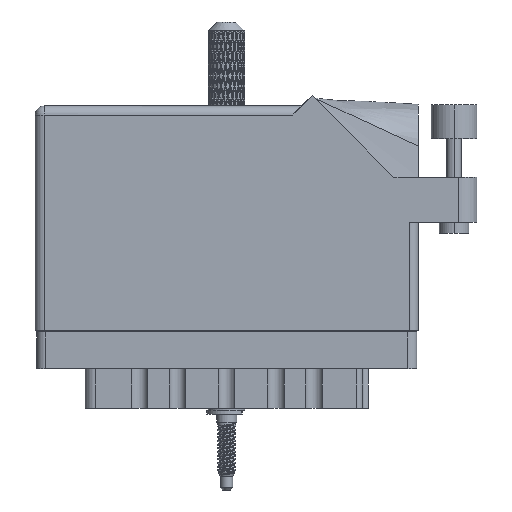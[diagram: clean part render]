
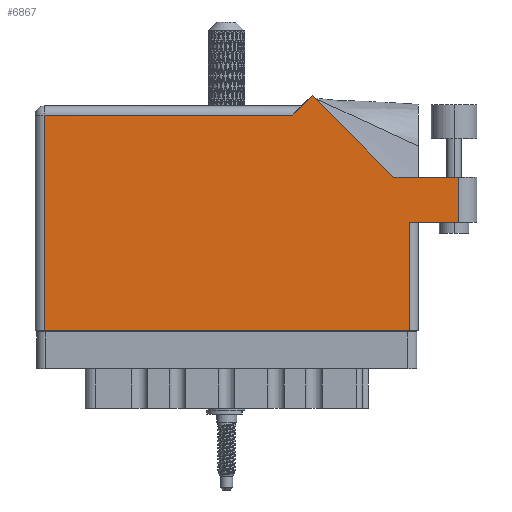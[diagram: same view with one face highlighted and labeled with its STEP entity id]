
A CAD part, front view. The second image highlights one B-rep face of the part: STEP entity #6867.
In plain terms, the highlighted face is planar.
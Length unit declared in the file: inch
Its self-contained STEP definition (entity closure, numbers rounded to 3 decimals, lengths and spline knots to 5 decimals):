
#557 = VERTEX_POINT ( 'NONE', #68809 ) ;
#1133 = CARTESIAN_POINT ( 'NONE',  ( 2.887, 0.737, 0. ) ) ;
#1200 = VECTOR ( 'NONE', #70098, 39.37008 ) ;
#2362 = LINE ( 'NONE', #81924, #64410 ) ;
#4994 = CARTESIAN_POINT ( 'NONE',  ( 0.062, 0., 0. ) ) ;
#5042 = CARTESIAN_POINT ( 'NONE',  ( 0.062, 0., 0. ) ) ;
#6867 = ADVANCED_FACE ( 'NONE', ( #55155 ), #33903, .F. ) ;
#9447 = DIRECTION ( 'NONE',  ( 0., 1., 0. ) ) ;
#10161 = LINE ( 'NONE', #42525, #63592 ) ;
#11218 = CARTESIAN_POINT ( 'NONE',  ( 1.757, 1.468, 0. ) ) ;
#14084 = EDGE_CURVE ( 'NONE', #20176, #74270, #48795, .T. ) ;
#15552 = VERTEX_POINT ( 'NONE', #52664 ) ;
#16435 = VECTOR ( 'NONE', #65704, 39.37008 ) ;
#17283 = CARTESIAN_POINT ( 'NONE',  ( 0., 1.53, 0. ) ) ;
#18609 = ORIENTED_EDGE ( 'NONE', *, *, #99939, .T. ) ;
#20176 = VERTEX_POINT ( 'NONE', #67402 ) ;
#20765 = VERTEX_POINT ( 'NONE', #1133 ) ;
#20951 = CARTESIAN_POINT ( 'NONE',  ( 0., 0., 0. ) ) ;
#24599 = DIRECTION ( 'NONE',  ( 0., 0., -1. ) ) ;
#25157 = LINE ( 'NONE', #73787, #16435 ) ;
#25183 = CARTESIAN_POINT ( 'NONE',  ( 2.44642, 1.044, 0. ) ) ;
#29127 = VERTEX_POINT ( 'NONE', #5042 ) ;
#30946 = EDGE_CURVE ( 'NONE', #44395, #58241, #56891, .T. ) ;
#31161 = EDGE_CURVE ( 'NONE', #58241, #20176, #25157, .T. ) ;
#33903 = PLANE ( 'NONE',  #53400 ) ;
#34952 = EDGE_CURVE ( 'NONE', #42357, #557, #43211, .T. ) ;
#35495 = DIRECTION ( 'NONE',  ( -1., 0., 0. ) ) ;
#35836 = ORIENTED_EDGE ( 'NONE', *, *, #30946, .T. ) ;
#37892 = ORIENTED_EDGE ( 'NONE', *, *, #34952, .T. ) ;
#39617 = ORIENTED_EDGE ( 'NONE', *, *, #91272, .T. ) ;
#41039 = VECTOR ( 'NONE', #79289, 39.37008 ) ;
#42357 = VERTEX_POINT ( 'NONE', #68161 ) ;
#42525 = CARTESIAN_POINT ( 'NONE',  ( 0., 1.468, 0. ) ) ;
#42828 = VECTOR ( 'NONE', #85472, 39.37008 ) ;
#43211 = LINE ( 'NONE', #64744, #116582 ) ;
#43825 = EDGE_CURVE ( 'NONE', #15552, #29127, #85927, .T. ) ;
#44395 = VERTEX_POINT ( 'NONE', #85089 ) ;
#48795 = LINE ( 'NONE', #68130, #1200 ) ;
#52664 = CARTESIAN_POINT ( 'NONE',  ( 0.062, 1.468, 0. ) ) ;
#53400 = AXIS2_PLACEMENT_3D ( 'NONE', #17283, #24599, #35495 ) ;
#54766 = EDGE_LOOP ( 'NONE', ( #62882, #92265, #35836, #59687, #82218, #18609, #77882, #39617, #37892 ) ) ;
#55155 = FACE_OUTER_BOUND ( 'NONE', #54766, .T. ) ;
#56891 = LINE ( 'NONE', #112990, #41039 ) ;
#58241 = VERTEX_POINT ( 'NONE', #25183 ) ;
#59687 = ORIENTED_EDGE ( 'NONE', *, *, #31161, .T. ) ;
#62882 = ORIENTED_EDGE ( 'NONE', *, *, #66747, .T. ) ;
#63592 = VECTOR ( 'NONE', #79992, 39.37008 ) ;
#64410 = VECTOR ( 'NONE', #91127, 39.37008 ) ;
#64744 = CARTESIAN_POINT ( 'NONE',  ( 2.55, 0.737, 0. ) ) ;
#65704 = DIRECTION ( 'NONE',  ( -0.707, 0.707, 0. ) ) ;
#66747 = EDGE_CURVE ( 'NONE', #557, #20765, #95709, .T. ) ;
#67258 = VECTOR ( 'NONE', #71187, 39.37008 ) ;
#67402 = CARTESIAN_POINT ( 'NONE',  ( 1.88971, 1.60071, 0. ) ) ;
#68130 = CARTESIAN_POINT ( 'NONE',  ( 1.819, 1.53, 0. ) ) ;
#68161 = CARTESIAN_POINT ( 'NONE',  ( 2.55, 0., 0. ) ) ;
#68809 = CARTESIAN_POINT ( 'NONE',  ( 2.55, 0.737, 0. ) ) ;
#70098 = DIRECTION ( 'NONE',  ( -0.707, -0.707, 0. ) ) ;
#71187 = DIRECTION ( 'NONE',  ( 0., -1., 0. ) ) ;
#73787 = CARTESIAN_POINT ( 'NONE',  ( 2.44642, 1.044, 0. ) ) ;
#74270 = VERTEX_POINT ( 'NONE', #11218 ) ;
#77882 = ORIENTED_EDGE ( 'NONE', *, *, #43825, .T. ) ;
#79289 = DIRECTION ( 'NONE',  ( -1., 0., 0. ) ) ;
#79992 = DIRECTION ( 'NONE',  ( -1., 0., 0. ) ) ;
#81924 = CARTESIAN_POINT ( 'NONE',  ( 2.887, 1.044, 0. ) ) ;
#82218 = ORIENTED_EDGE ( 'NONE', *, *, #14084, .T. ) ;
#85089 = CARTESIAN_POINT ( 'NONE',  ( 2.887, 1.044, 0. ) ) ;
#85472 = DIRECTION ( 'NONE',  ( 1., 0., 0. ) ) ;
#85927 = LINE ( 'NONE', #4994, #67258 ) ;
#90935 = EDGE_CURVE ( 'NONE', #20765, #44395, #2362, .T. ) ;
#91127 = DIRECTION ( 'NONE',  ( 0., 1., 0. ) ) ;
#91272 = EDGE_CURVE ( 'NONE', #29127, #42357, #116220, .T. ) ;
#92265 = ORIENTED_EDGE ( 'NONE', *, *, #90935, .T. ) ;
#92839 = VECTOR ( 'NONE', #111563, 39.37008 ) ;
#95709 = LINE ( 'NONE', #103094, #92839 ) ;
#99939 = EDGE_CURVE ( 'NONE', #74270, #15552, #10161, .T. ) ;
#103094 = CARTESIAN_POINT ( 'NONE',  ( 2.612, 0.737, 0. ) ) ;
#111563 = DIRECTION ( 'NONE',  ( 1., 0., 0. ) ) ;
#112990 = CARTESIAN_POINT ( 'NONE',  ( 3.012, 1.044, 0. ) ) ;
#116220 = LINE ( 'NONE', #20951, #42828 ) ;
#116582 = VECTOR ( 'NONE', #9447, 39.37008 ) ;
